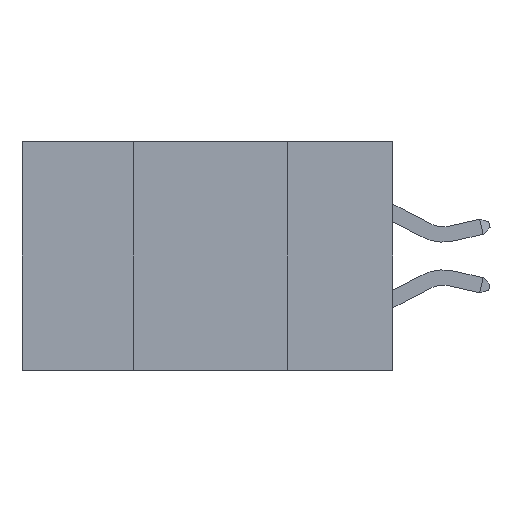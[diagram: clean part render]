
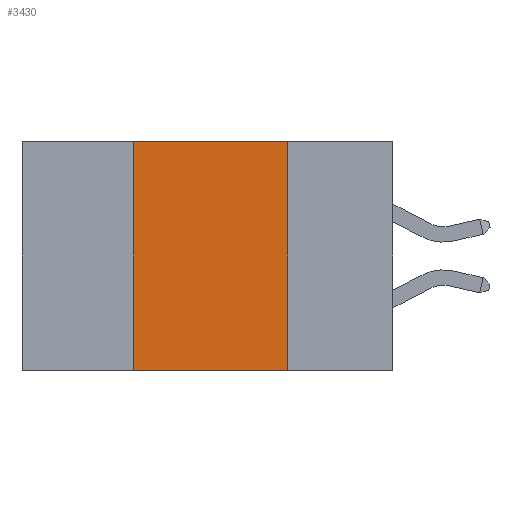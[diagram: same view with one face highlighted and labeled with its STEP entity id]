
A CAD part, left-side view. The second image highlights one B-rep face of the part: STEP entity #3430.
In plain terms, the highlighted planar face has unit normal (-1, 0, 0).
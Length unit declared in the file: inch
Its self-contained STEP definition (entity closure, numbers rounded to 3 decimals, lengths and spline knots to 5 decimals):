
#702 = CARTESIAN_POINT ( 'NONE',  ( 0., 0.42, 0. ) ) ;
#3430 = ADVANCED_FACE ( 'NONE', ( #19975 ), #4301, .F. ) ;
#4112 = DIRECTION ( 'NONE',  ( 1., 0., 0. ) ) ;
#4301 = PLANE ( 'NONE',  #30706 ) ;
#4950 = VECTOR ( 'NONE', #18467, 39.37008 ) ;
#6864 = ORIENTED_EDGE ( 'NONE', *, *, #39016, .T. ) ;
#7125 = CARTESIAN_POINT ( 'NONE',  ( 0., 0.17, 0. ) ) ;
#10089 = CARTESIAN_POINT ( 'NONE',  ( 0., 0.17, 0. ) ) ;
#12331 = EDGE_CURVE ( 'NONE', #36644, #16525, #19645, .T. ) ;
#12873 = EDGE_LOOP ( 'NONE', ( #14259, #15222, #31213, #6864 ) ) ;
#14259 = ORIENTED_EDGE ( 'NONE', *, *, #23535, .F. ) ;
#15222 = ORIENTED_EDGE ( 'NONE', *, *, #27012, .F. ) ;
#16324 = CARTESIAN_POINT ( 'NONE',  ( 0., 0.6, 0. ) ) ;
#16404 = DIRECTION ( 'NONE',  ( 0., 0., -1. ) ) ;
#16525 = VERTEX_POINT ( 'NONE', #21137 ) ;
#16928 = DIRECTION ( 'NONE',  ( 0., 0., -1. ) ) ;
#18467 = DIRECTION ( 'NONE',  ( 0., -1., 0. ) ) ;
#19645 = LINE ( 'NONE', #702, #21302 ) ;
#19975 = FACE_OUTER_BOUND ( 'NONE', #12873, .T. ) ;
#21015 = LINE ( 'NONE', #36517, #37060 ) ;
#21137 = CARTESIAN_POINT ( 'NONE',  ( 0., 0.42, 0. ) ) ;
#21302 = VECTOR ( 'NONE', #28020, 39.37008 ) ;
#21669 = VERTEX_POINT ( 'NONE', #25769 ) ;
#23535 = EDGE_CURVE ( 'NONE', #35966, #21669, #32865, .T. ) ;
#24066 = DIRECTION ( 'NONE',  ( 0., -1., 0. ) ) ;
#25769 = CARTESIAN_POINT ( 'NONE',  ( 0., 0.17, -0.37 ) ) ;
#27012 = EDGE_CURVE ( 'NONE', #16525, #35966, #21015, .T. ) ;
#27650 = LINE ( 'NONE', #34164, #4950 ) ;
#28020 = DIRECTION ( 'NONE',  ( 0., 0., 1. ) ) ;
#30334 = VECTOR ( 'NONE', #16404, 39.37008 ) ;
#30706 = AXIS2_PLACEMENT_3D ( 'NONE', #16324, #4112, #16928 ) ;
#30839 = CARTESIAN_POINT ( 'NONE',  ( 0., 0.42, -0.37 ) ) ;
#31213 = ORIENTED_EDGE ( 'NONE', *, *, #12331, .F. ) ;
#32865 = LINE ( 'NONE', #10089, #30334 ) ;
#34164 = CARTESIAN_POINT ( 'NONE',  ( 0., 0.6, -0.37 ) ) ;
#35966 = VERTEX_POINT ( 'NONE', #7125 ) ;
#36517 = CARTESIAN_POINT ( 'NONE',  ( 0., 0.6, 0. ) ) ;
#36644 = VERTEX_POINT ( 'NONE', #30839 ) ;
#37060 = VECTOR ( 'NONE', #24066, 39.37008 ) ;
#39016 = EDGE_CURVE ( 'NONE', #36644, #21669, #27650, .T. ) ;
